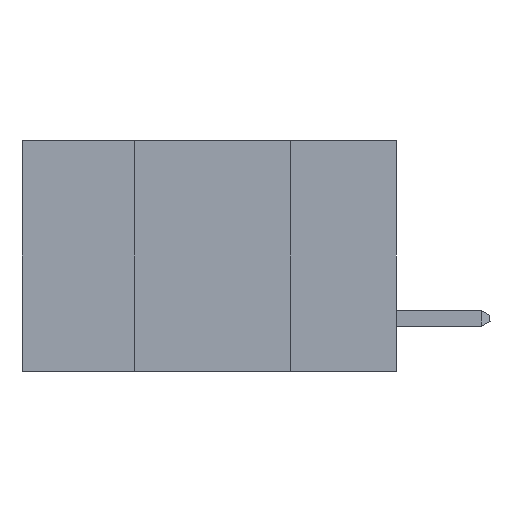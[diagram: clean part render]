
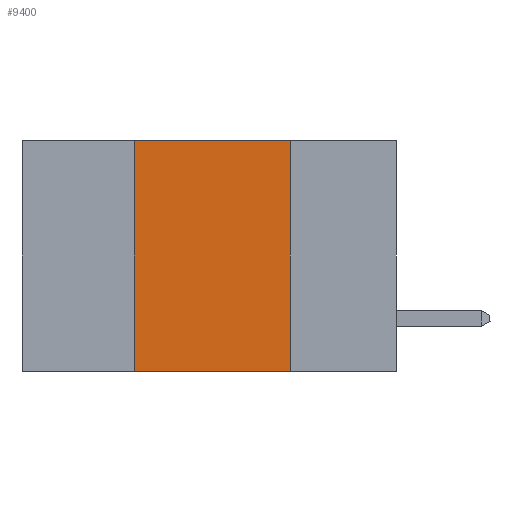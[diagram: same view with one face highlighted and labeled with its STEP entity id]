
A CAD part, left-side view. The second image highlights one B-rep face of the part: STEP entity #9400.
In plain terms, the highlighted planar face has unit normal (-1, 0, 0).
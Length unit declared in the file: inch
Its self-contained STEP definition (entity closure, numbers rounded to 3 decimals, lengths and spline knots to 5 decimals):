
#114 = DIRECTION ( 'NONE',  ( 0., 0., 1. ) ) ;
#718 = DIRECTION ( 'NONE',  ( 0., 0., -1. ) ) ;
#1194 = AXIS2_PLACEMENT_3D ( 'NONE', #3164, #3060, #3038 ) ;
#2090 = VERTEX_POINT ( 'NONE', #16141 ) ;
#2415 = CARTESIAN_POINT ( 'NONE',  ( 0., 0.42, -0.37 ) ) ;
#3038 = DIRECTION ( 'NONE',  ( 0., 0., -1. ) ) ;
#3060 = DIRECTION ( 'NONE',  ( 1., 0., 0. ) ) ;
#3164 = CARTESIAN_POINT ( 'NONE',  ( 0., 0.6, 0. ) ) ;
#3545 = PLANE ( 'NONE',  #1194 ) ;
#3608 = CARTESIAN_POINT ( 'NONE',  ( 0., 0.6, 0. ) ) ;
#3811 = VERTEX_POINT ( 'NONE', #2415 ) ;
#4039 = VECTOR ( 'NONE', #718, 39.37008 ) ;
#4432 = ORIENTED_EDGE ( 'NONE', *, *, #13987, .F. ) ;
#5354 = DIRECTION ( 'NONE',  ( 0., -1., 0. ) ) ;
#6349 = DIRECTION ( 'NONE',  ( 0., -1., 0. ) ) ;
#6354 = ORIENTED_EDGE ( 'NONE', *, *, #21713, .F. ) ;
#7131 = CARTESIAN_POINT ( 'NONE',  ( 0., 0.6, -0.37 ) ) ;
#7188 = ORIENTED_EDGE ( 'NONE', *, *, #11193, .T. ) ;
#7306 = FACE_OUTER_BOUND ( 'NONE', #20882, .T. ) ;
#7579 = LINE ( 'NONE', #21255, #4039 ) ;
#8249 = LINE ( 'NONE', #3608, #16943 ) ;
#8846 = VERTEX_POINT ( 'NONE', #19403 ) ;
#9400 = ADVANCED_FACE ( 'NONE', ( #7306 ), #3545, .F. ) ;
#11193 = EDGE_CURVE ( 'NONE', #3811, #8846, #16027, .T. ) ;
#12555 = VERTEX_POINT ( 'NONE', #17290 ) ;
#13987 = EDGE_CURVE ( 'NONE', #3811, #12555, #20349, .T. ) ;
#15916 = VECTOR ( 'NONE', #114, 39.37008 ) ;
#16027 = LINE ( 'NONE', #7131, #19461 ) ;
#16141 = CARTESIAN_POINT ( 'NONE',  ( 0., 0.17, 0. ) ) ;
#16943 = VECTOR ( 'NONE', #5354, 39.37008 ) ;
#17290 = CARTESIAN_POINT ( 'NONE',  ( 0., 0.42, 0. ) ) ;
#17379 = CARTESIAN_POINT ( 'NONE',  ( 0., 0.42, 0. ) ) ;
#19403 = CARTESIAN_POINT ( 'NONE',  ( 0., 0.17, -0.37 ) ) ;
#19461 = VECTOR ( 'NONE', #6349, 39.37008 ) ;
#19866 = EDGE_CURVE ( 'NONE', #2090, #8846, #7579, .T. ) ;
#20349 = LINE ( 'NONE', #17379, #15916 ) ;
#20504 = ORIENTED_EDGE ( 'NONE', *, *, #19866, .F. ) ;
#20882 = EDGE_LOOP ( 'NONE', ( #20504, #6354, #4432, #7188 ) ) ;
#21255 = CARTESIAN_POINT ( 'NONE',  ( 0., 0.17, 0. ) ) ;
#21713 = EDGE_CURVE ( 'NONE', #12555, #2090, #8249, .T. ) ;
